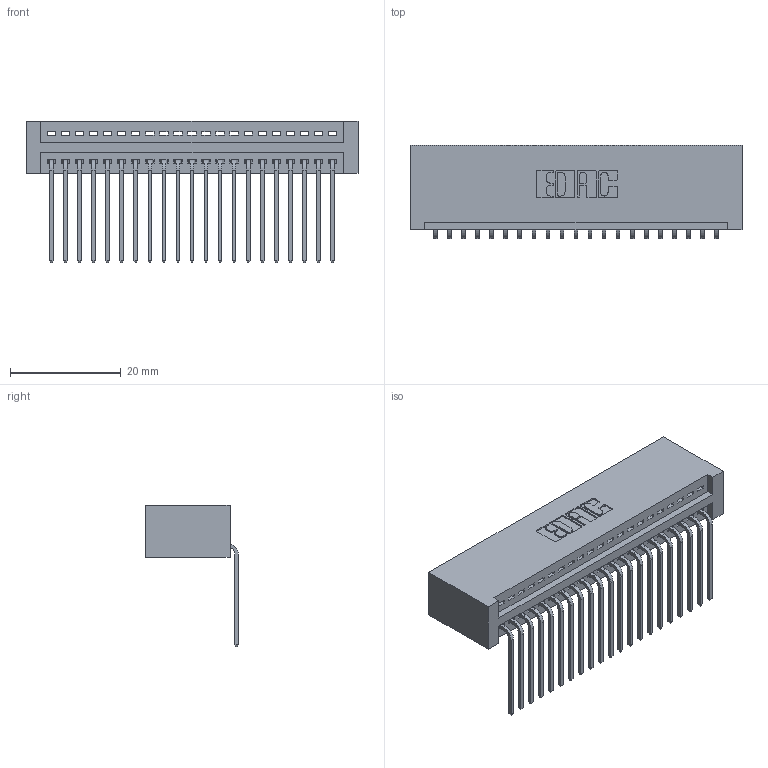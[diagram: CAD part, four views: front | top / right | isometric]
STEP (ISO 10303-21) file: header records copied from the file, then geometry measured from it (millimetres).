
FILE_DESCRIPTION (( 'STEP AP203' ), '1' );
FILE_NAME ('345-021-559-101.STEP', '2018-08-20T10:14:01', ( '' ), ( '' ), 'SwSTEP 2.0', 'SolidWorks 2016', '' );
FILE_SCHEMA (( 'CONFIG_CONTROL_DESIGN' ));
Length unit declared in the file: inch
Products named in the file (3): 345-292-001_558 559 Tail - 1; 345-021-559-101; 345 Part_No Mounting Lugs
Assembly tree (22 placements, depth 2):
  345-021-559-101
    345 Part_No Mounting Lugs
    345-292-001_558 559 Tail - 1  x21
Bounding box: 59.94 x 16.75 x 25.53 mm (x, y, z)
Volume: 6175.8 mm3; surface area: 8523 mm2
Topology: 22 solids, 22 shells, 1378 faces, 4139 edges, 2730 vertices
Faces by surface type: plane 958, cylinder 420
Entity records: 18439 total; most frequent: CARTESIAN_POINT 3203, ORIENTED_EDGE 3158, DIRECTION 2821, EDGE_CURVE 1579, LINE 1371, VECTOR 1371, VERTEX_POINT 1050, AXIS2_PLACEMENT_3D 725
